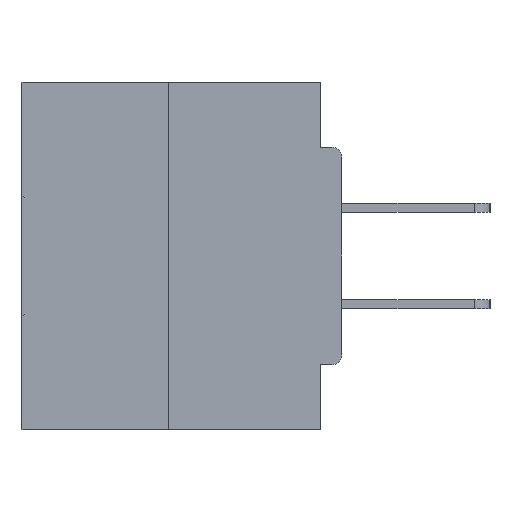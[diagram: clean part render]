
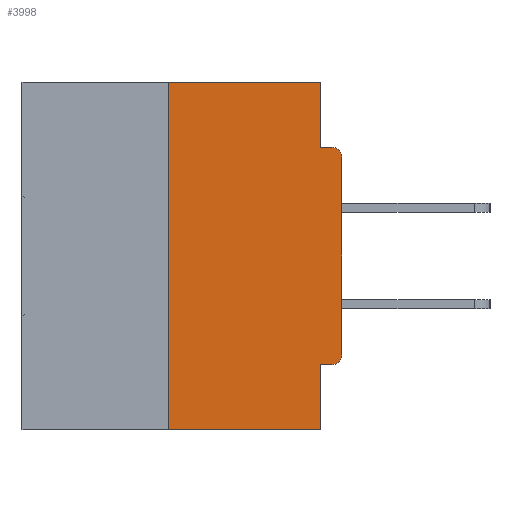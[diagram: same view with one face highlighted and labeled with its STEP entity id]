
A CAD part, left-side view. The second image highlights one B-rep face of the part: STEP entity #3998.
In plain terms, the highlighted planar face has unit normal (-1, 0, 0).
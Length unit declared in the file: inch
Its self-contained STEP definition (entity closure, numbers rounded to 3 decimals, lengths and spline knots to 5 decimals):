
#149 = CARTESIAN_POINT ( 'NONE',  ( 0., 0.25, 0. ) ) ;
#718 = EDGE_LOOP ( 'NONE', ( #14168, #35745, #27532, #23193, #5317, #2818, #9202, #34444, #34594, #7710 ) ) ;
#1594 = LINE ( 'NONE', #7279, #31260 ) ;
#2171 = AXIS2_PLACEMENT_3D ( 'NONE', #22025, #2682, #12367 ) ;
#2422 = VERTEX_POINT ( 'NONE', #20867 ) ;
#2682 = DIRECTION ( 'NONE',  ( -1., 0., 0. ) ) ;
#2818 = ORIENTED_EDGE ( 'NONE', *, *, #13662, .T. ) ;
#2923 = DIRECTION ( 'NONE',  ( 0., -1., 0. ) ) ;
#3998 = ADVANCED_FACE ( 'NONE', ( #37524 ), #26841, .F. ) ;
#4023 = VERTEX_POINT ( 'NONE', #13309 ) ;
#5242 = LINE ( 'NONE', #36051, #11691 ) ;
#5317 = ORIENTED_EDGE ( 'NONE', *, *, #12849, .F. ) ;
#5968 = CIRCLE ( 'NONE', #8196, 0.015 ) ;
#6359 = LINE ( 'NONE', #26989, #17769 ) ;
#7279 = CARTESIAN_POINT ( 'NONE',  ( 0., 0., 0. ) ) ;
#7710 = ORIENTED_EDGE ( 'NONE', *, *, #7831, .F. ) ;
#7831 = EDGE_CURVE ( 'NONE', #4023, #38816, #29468, .T. ) ;
#7929 = CARTESIAN_POINT ( 'NONE',  ( 0., 0.46, 0. ) ) ;
#7958 = DIRECTION ( 'NONE',  ( 0., 0., -1. ) ) ;
#8196 = AXIS2_PLACEMENT_3D ( 'NONE', #34337, #33913, #18614 ) ;
#8199 = CARTESIAN_POINT ( 'NONE',  ( 0., 0.015, -0.4065 ) ) ;
#8607 = DIRECTION ( 'NONE',  ( 0., 1., 0. ) ) ;
#8950 = EDGE_CURVE ( 'NONE', #11026, #4023, #5242, .T. ) ;
#8965 = CARTESIAN_POINT ( 'NONE',  ( 0., 0.031, -0.5 ) ) ;
#9016 = VERTEX_POINT ( 'NONE', #11339 ) ;
#9157 = CARTESIAN_POINT ( 'NONE',  ( 0., 0., -0.0935 ) ) ;
#9202 = ORIENTED_EDGE ( 'NONE', *, *, #17649, .T. ) ;
#9794 = CARTESIAN_POINT ( 'NONE',  ( 0., 0.25, -0.5 ) ) ;
#9865 = VECTOR ( 'NONE', #30552, 39.37008 ) ;
#11026 = VERTEX_POINT ( 'NONE', #149 ) ;
#11249 = EDGE_CURVE ( 'NONE', #38816, #19659, #33250, .T. ) ;
#11339 = CARTESIAN_POINT ( 'NONE',  ( 0., 0., -0.1085 ) ) ;
#11430 = CARTESIAN_POINT ( 'NONE',  ( 0., 0.031, 0. ) ) ;
#11691 = VECTOR ( 'NONE', #23757, 39.37008 ) ;
#12367 = DIRECTION ( 'NONE',  ( 0., 0., -1. ) ) ;
#12849 = EDGE_CURVE ( 'NONE', #33237, #30910, #21795, .T. ) ;
#13309 = CARTESIAN_POINT ( 'NONE',  ( 0., 0.031, 0. ) ) ;
#13662 = EDGE_CURVE ( 'NONE', #33237, #33626, #25686, .T. ) ;
#14168 = ORIENTED_EDGE ( 'NONE', *, *, #8950, .F. ) ;
#14963 = CARTESIAN_POINT ( 'NONE',  ( 0., 0.031, -0.4065 ) ) ;
#16152 = CARTESIAN_POINT ( 'NONE',  ( 0., 0., -0.3915 ) ) ;
#17289 = EDGE_CURVE ( 'NONE', #30910, #2422, #37168, .T. ) ;
#17649 = EDGE_CURVE ( 'NONE', #33626, #9016, #1594, .T. ) ;
#17769 = VECTOR ( 'NONE', #21059, 39.37008 ) ;
#17954 = CARTESIAN_POINT ( 'NONE',  ( 0., 0.031, -0.0935 ) ) ;
#18614 = DIRECTION ( 'NONE',  ( 0., 0., -1. ) ) ;
#19336 = EDGE_CURVE ( 'NONE', #9016, #19659, #5968, .T. ) ;
#19659 = VERTEX_POINT ( 'NONE', #23299 ) ;
#19900 = AXIS2_PLACEMENT_3D ( 'NONE', #7929, #39553, #30067 ) ;
#20199 = EDGE_CURVE ( 'NONE', #40504, #11026, #36037, .T. ) ;
#20864 = CARTESIAN_POINT ( 'NONE',  ( 0., 0.25, 0. ) ) ;
#20867 = CARTESIAN_POINT ( 'NONE',  ( 0., 0.031, -0.5 ) ) ;
#21059 = DIRECTION ( 'NONE',  ( 0., -1., 0. ) ) ;
#21709 = CARTESIAN_POINT ( 'NONE',  ( 0., 0., -0.4065 ) ) ;
#21795 = LINE ( 'NONE', #21709, #28214 ) ;
#22025 = CARTESIAN_POINT ( 'NONE',  ( 0., 0.015, -0.3915 ) ) ;
#22402 = VECTOR ( 'NONE', #2923, 39.37008 ) ;
#22763 = DIRECTION ( 'NONE',  ( 0., 0., 1. ) ) ;
#23193 = ORIENTED_EDGE ( 'NONE', *, *, #17289, .F. ) ;
#23299 = CARTESIAN_POINT ( 'NONE',  ( 0., 0.015, -0.0935 ) ) ;
#23757 = DIRECTION ( 'NONE',  ( 0., -1., 0. ) ) ;
#25686 = CIRCLE ( 'NONE', #2171, 0.015 ) ;
#26841 = PLANE ( 'NONE',  #19900 ) ;
#26989 = CARTESIAN_POINT ( 'NONE',  ( 0., 0.46, -0.5 ) ) ;
#27532 = ORIENTED_EDGE ( 'NONE', *, *, #30890, .T. ) ;
#28214 = VECTOR ( 'NONE', #8607, 39.37008 ) ;
#29468 = LINE ( 'NONE', #11430, #32889 ) ;
#30067 = DIRECTION ( 'NONE',  ( 0., 0., -1. ) ) ;
#30552 = DIRECTION ( 'NONE',  ( 0., 0., 1. ) ) ;
#30890 = EDGE_CURVE ( 'NONE', #40504, #2422, #6359, .T. ) ;
#30910 = VERTEX_POINT ( 'NONE', #14963 ) ;
#31260 = VECTOR ( 'NONE', #22763, 39.37008 ) ;
#32889 = VECTOR ( 'NONE', #7958, 39.37008 ) ;
#33237 = VERTEX_POINT ( 'NONE', #8199 ) ;
#33250 = LINE ( 'NONE', #9157, #22402 ) ;
#33626 = VERTEX_POINT ( 'NONE', #16152 ) ;
#33913 = DIRECTION ( 'NONE',  ( -1., 0., 0. ) ) ;
#34253 = DIRECTION ( 'NONE',  ( 0., 0., -1. ) ) ;
#34337 = CARTESIAN_POINT ( 'NONE',  ( 0., 0.015, -0.1085 ) ) ;
#34444 = ORIENTED_EDGE ( 'NONE', *, *, #19336, .T. ) ;
#34594 = ORIENTED_EDGE ( 'NONE', *, *, #11249, .F. ) ;
#35745 = ORIENTED_EDGE ( 'NONE', *, *, #20199, .F. ) ;
#36037 = LINE ( 'NONE', #20864, #9865 ) ;
#36051 = CARTESIAN_POINT ( 'NONE',  ( 0., 0.46, 0. ) ) ;
#37168 = LINE ( 'NONE', #8965, #40635 ) ;
#37524 = FACE_OUTER_BOUND ( 'NONE', #718, .T. ) ;
#38816 = VERTEX_POINT ( 'NONE', #17954 ) ;
#39553 = DIRECTION ( 'NONE',  ( 1., 0., 0. ) ) ;
#40504 = VERTEX_POINT ( 'NONE', #9794 ) ;
#40635 = VECTOR ( 'NONE', #34253, 39.37008 ) ;
